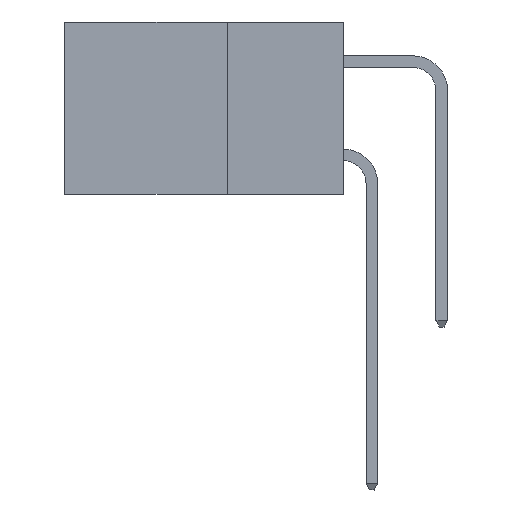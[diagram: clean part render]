
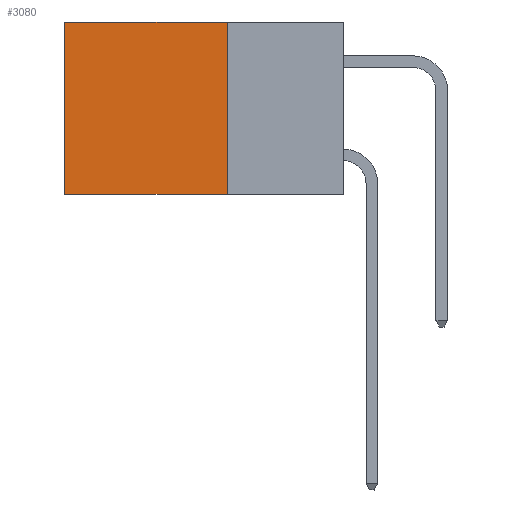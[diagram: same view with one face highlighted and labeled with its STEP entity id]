
A CAD part, left-side view. The second image highlights one B-rep face of the part: STEP entity #3080.
In plain terms, the highlighted planar face has unit normal (-1, 0, 0).
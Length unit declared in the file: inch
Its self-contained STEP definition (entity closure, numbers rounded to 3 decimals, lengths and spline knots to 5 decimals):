
#4 = VECTOR ( 'NONE', #8296, 39.37008 ) ;
#1096 = VERTEX_POINT ( 'NONE', #4103 ) ;
#1343 = VECTOR ( 'NONE', #12425, 39.37008 ) ;
#1385 = CARTESIAN_POINT ( 'NONE',  ( 0.2615, 0.6, -0.37 ) ) ;
#1464 = LINE ( 'NONE', #9458, #5759 ) ;
#1529 = PLANE ( 'NONE',  #12409 ) ;
#2265 = DIRECTION ( 'NONE',  ( 0., 1., 0. ) ) ;
#2327 = VERTEX_POINT ( 'NONE', #11254 ) ;
#3026 = CARTESIAN_POINT ( 'NONE',  ( 0.2615, 0.25, -0.37 ) ) ;
#3080 = ADVANCED_FACE ( 'NONE', ( #11841 ), #1529, .F. ) ;
#3089 = LINE ( 'NONE', #3026, #4 ) ;
#4000 = DIRECTION ( 'NONE',  ( 0., 1., 0. ) ) ;
#4103 = CARTESIAN_POINT ( 'NONE',  ( 0.2615, 0.6, -0.37 ) ) ;
#4137 = EDGE_CURVE ( 'NONE', #2327, #9231, #3089, .T. ) ;
#4508 = CARTESIAN_POINT ( 'NONE',  ( 0.2615, 0.25, -0.37 ) ) ;
#5553 = DIRECTION ( 'NONE',  ( 0., 0., -1. ) ) ;
#5569 = VECTOR ( 'NONE', #4000, 39.37008 ) ;
#5743 = ORIENTED_EDGE ( 'NONE', *, *, #4137, .F. ) ;
#5759 = VECTOR ( 'NONE', #2265, 39.37008 ) ;
#6959 = LINE ( 'NONE', #11258, #5569 ) ;
#7939 = ORIENTED_EDGE ( 'NONE', *, *, #7971, .T. ) ;
#7971 = EDGE_CURVE ( 'NONE', #8475, #1096, #12556, .T. ) ;
#8296 = DIRECTION ( 'NONE',  ( 0., 0., -1. ) ) ;
#8462 = ORIENTED_EDGE ( 'NONE', *, *, #13047, .T. ) ;
#8475 = VERTEX_POINT ( 'NONE', #11422 ) ;
#9231 = VERTEX_POINT ( 'NONE', #10259 ) ;
#9336 = ORIENTED_EDGE ( 'NONE', *, *, #11837, .F. ) ;
#9458 = CARTESIAN_POINT ( 'NONE',  ( 0.2615, 0.25, -0.37 ) ) ;
#10259 = CARTESIAN_POINT ( 'NONE',  ( 0.2615, 0.25, -0.37 ) ) ;
#10515 = DIRECTION ( 'NONE',  ( 1., 0., 0. ) ) ;
#11254 = CARTESIAN_POINT ( 'NONE',  ( 0.2615, 0.25, 0. ) ) ;
#11258 = CARTESIAN_POINT ( 'NONE',  ( 0.2615, 0.25, 0. ) ) ;
#11422 = CARTESIAN_POINT ( 'NONE',  ( 0.2615, 0.6, 0. ) ) ;
#11837 = EDGE_CURVE ( 'NONE', #9231, #1096, #1464, .T. ) ;
#11841 = FACE_OUTER_BOUND ( 'NONE', #12037, .T. ) ;
#12037 = EDGE_LOOP ( 'NONE', ( #7939, #9336, #5743, #8462 ) ) ;
#12409 = AXIS2_PLACEMENT_3D ( 'NONE', #4508, #10515, #5553 ) ;
#12425 = DIRECTION ( 'NONE',  ( 0., 0., -1. ) ) ;
#12556 = LINE ( 'NONE', #1385, #1343 ) ;
#13047 = EDGE_CURVE ( 'NONE', #2327, #8475, #6959, .T. ) ;
